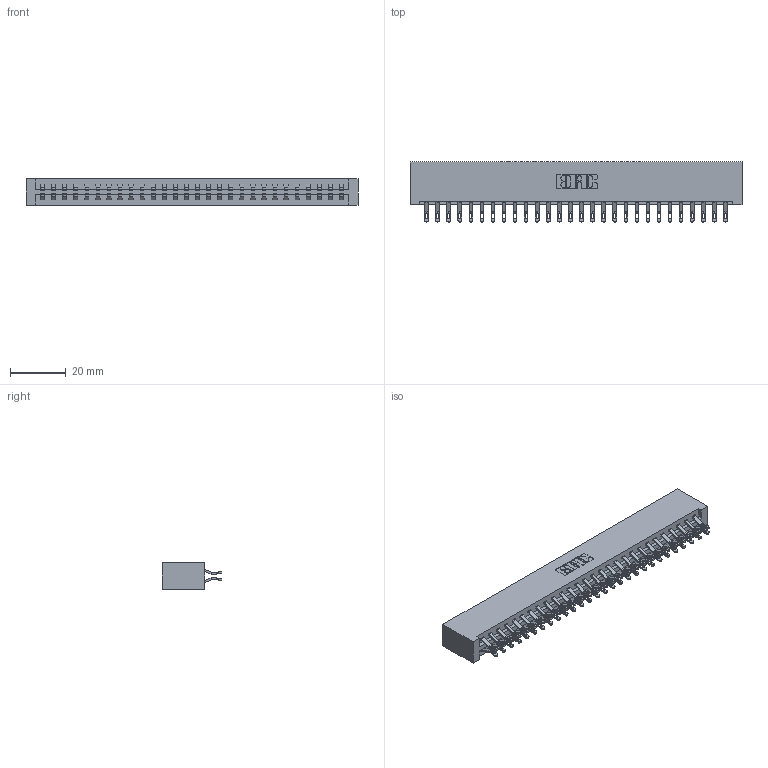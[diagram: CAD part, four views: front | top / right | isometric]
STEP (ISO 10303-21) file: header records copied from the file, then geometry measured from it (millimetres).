
FILE_DESCRIPTION (( 'STEP AP203' ), '1' );
FILE_NAME ('387-056-555-201.STEP', '2018-09-21T00:11:13', ( '' ), ( '' ), 'SwSTEP 2.0', 'SolidWorks 2016', '' );
FILE_SCHEMA (( 'CONFIG_CONTROL_DESIGN' ));
Length unit declared in the file: inch
Products named in the file (3): 387-056-555-201; 337 Part_No Mounting Lugs; 345-292-001_555 Tail
Assembly tree (57 placements, depth 2):
  387-056-555-201
    337 Part_No Mounting Lugs
    345-292-001_555 Tail  x56
Bounding box: 118.82 x 21.47 x 9.4 mm (x, y, z)
Volume: 13259.1 mm3; surface area: 15521.7 mm2
Topology: 57 solids, 57 shells, 3466 faces, 10871 edges, 7246 vertices
Faces by surface type: plane 2082, cylinder 1384
Entity records: 23569 total; most frequent: CARTESIAN_POINT 4016, ORIENTED_EDGE 3922, DIRECTION 3405, EDGE_CURVE 1961, VECTOR 1821, LINE 1821, VERTEX_POINT 1306, AXIS2_PLACEMENT_3D 792
